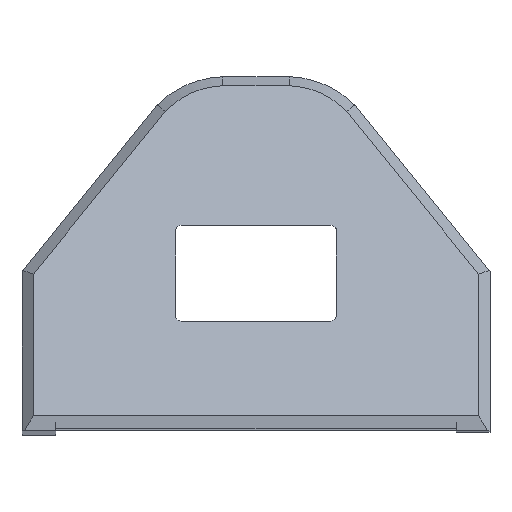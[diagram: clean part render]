
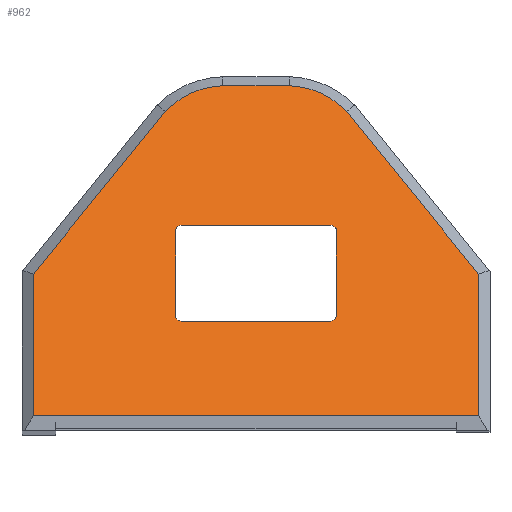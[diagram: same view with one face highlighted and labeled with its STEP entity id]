
A CAD part, top view. The second image highlights one B-rep face of the part: STEP entity #962.
In plain terms, the highlighted planar face has unit normal (0, 0.603, 0.798).
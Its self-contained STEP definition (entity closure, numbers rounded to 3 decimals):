
#20=FACE_BOUND('',#347,.T.);
#38=PLANE('',#1056);
#68=ELLIPSE('',#1057,0.626,0.5);
#69=ELLIPSE('',#1058,0.626,0.5);
#70=ELLIPSE('',#1059,0.626,0.5);
#71=ELLIPSE('',#1060,0.626,0.5);
#100=LINE('',#1491,#189);
#103=LINE('',#1498,#192);
#106=LINE('',#1529,#195);
#111=LINE('',#1589,#200);
#113=LINE('',#1665,#202);
#119=LINE('',#1677,#208);
#131=LINE('',#1705,#220);
#132=LINE('',#1709,#221);
#133=LINE('',#1713,#222);
#134=LINE('',#1717,#223);
#189=VECTOR('',#1193,10.);
#192=VECTOR('',#1198,10.);
#195=VECTOR('',#1205,10.);
#200=VECTOR('',#1212,10.);
#202=VECTOR('',#1216,10.);
#208=VECTOR('',#1228,10.);
#220=VECTOR('',#1252,10.);
#221=VECTOR('',#1255,10.);
#222=VECTOR('',#1258,10.);
#223=VECTOR('',#1261,10.);
#293=FACE_OUTER_BOUND('',#346,.T.);
#346=EDGE_LOOP('',(#794,#795,#796,#797,#798,#799,#800,#801));
#347=EDGE_LOOP('',(#802,#803,#804,#805,#806,#807,#808,#809));
#379=B_SPLINE_CURVE_WITH_KNOTS('',3,(#1558,#1559,#1560,#1561,#1562),
 .UNSPECIFIED.,.F.,.F.,(4,1,4),(-3.112,-2.672,-2.338),
 .UNSPECIFIED.);
#384=B_SPLINE_CURVE_WITH_KNOTS('',3,(#1626,#1627,#1628,#1629,#1630),
 .UNSPECIFIED.,.F.,.F.,(4,1,4),(2.338,2.783,3.112),
 .UNSPECIFIED.);
#446=VERTEX_POINT('',#1488);
#447=VERTEX_POINT('',#1490);
#449=VERTEX_POINT('',#1496);
#450=VERTEX_POINT('',#1497);
#454=VERTEX_POINT('',#1528);
#458=VERTEX_POINT('',#1557);
#461=VERTEX_POINT('',#1588);
#463=VERTEX_POINT('',#1625);
#477=VERTEX_POINT('',#1703);
#478=VERTEX_POINT('',#1704);
#479=VERTEX_POINT('',#1706);
#480=VERTEX_POINT('',#1708);
#481=VERTEX_POINT('',#1710);
#482=VERTEX_POINT('',#1712);
#483=VERTEX_POINT('',#1714);
#484=VERTEX_POINT('',#1716);
#554=EDGE_CURVE('',#446,#447,#100,.T.);
#557=EDGE_CURVE('',#449,#450,#103,.T.);
#562=EDGE_CURVE('',#450,#454,#106,.T.);
#567=EDGE_CURVE('',#458,#449,#379,.T.);
#571=EDGE_CURVE('',#461,#458,#111,.T.);
#574=EDGE_CURVE('',#463,#461,#384,.T.);
#578=EDGE_CURVE('',#447,#463,#113,.T.);
#585=EDGE_CURVE('',#454,#446,#119,.T.);
#598=EDGE_CURVE('',#477,#478,#131,.T.);
#599=EDGE_CURVE('',#478,#479,#68,.T.);
#600=EDGE_CURVE('',#479,#480,#132,.T.);
#601=EDGE_CURVE('',#480,#481,#69,.T.);
#602=EDGE_CURVE('',#481,#482,#133,.T.);
#603=EDGE_CURVE('',#482,#483,#70,.T.);
#604=EDGE_CURVE('',#483,#484,#134,.T.);
#605=EDGE_CURVE('',#484,#477,#71,.T.);
#794=ORIENTED_EDGE('',*,*,#554,.F.);
#795=ORIENTED_EDGE('',*,*,#585,.F.);
#796=ORIENTED_EDGE('',*,*,#562,.F.);
#797=ORIENTED_EDGE('',*,*,#557,.F.);
#798=ORIENTED_EDGE('',*,*,#567,.F.);
#799=ORIENTED_EDGE('',*,*,#571,.F.);
#800=ORIENTED_EDGE('',*,*,#574,.F.);
#801=ORIENTED_EDGE('',*,*,#578,.F.);
#802=ORIENTED_EDGE('',*,*,#598,.T.);
#803=ORIENTED_EDGE('',*,*,#599,.T.);
#804=ORIENTED_EDGE('',*,*,#600,.T.);
#805=ORIENTED_EDGE('',*,*,#601,.T.);
#806=ORIENTED_EDGE('',*,*,#602,.T.);
#807=ORIENTED_EDGE('',*,*,#603,.T.);
#808=ORIENTED_EDGE('',*,*,#604,.T.);
#809=ORIENTED_EDGE('',*,*,#605,.T.);
#962=ADVANCED_FACE('',(#293,#20),#38,.T.);
#1056=AXIS2_PLACEMENT_3D('',#1702,#1250,#1251);
#1057=AXIS2_PLACEMENT_3D('',#1707,#1253,#1254);
#1058=AXIS2_PLACEMENT_3D('',#1711,#1256,#1257);
#1059=AXIS2_PLACEMENT_3D('',#1715,#1259,#1260);
#1060=AXIS2_PLACEMENT_3D('',#1718,#1262,#1263);
#1193=DIRECTION('',(0.,0.798,-0.602));
#1198=DIRECTION('',(0.543,-0.67,0.506));
#1205=DIRECTION('',(0.,-0.798,0.602));
#1212=DIRECTION('',(1.,0.,0.));
#1216=DIRECTION('',(0.543,0.67,-0.506));
#1228=DIRECTION('',(-1.,0.,0.));
#1250=DIRECTION('center_axis',(0.,0.602,0.798));
#1251=DIRECTION('ref_axis',(1.,0.,0.));
#1252=DIRECTION('',(1.,0.,0.));
#1253=DIRECTION('center_axis',(0.,-0.602,-0.798));
#1254=DIRECTION('ref_axis',(0.,0.798,-0.602));
#1255=DIRECTION('',(0.,-0.798,0.602));
#1256=DIRECTION('center_axis',(0.,-0.602,-0.798));
#1257=DIRECTION('ref_axis',(0.,0.798,-0.602));
#1258=DIRECTION('',(-1.,0.,0.));
#1259=DIRECTION('center_axis',(0.,-0.602,-0.798));
#1260=DIRECTION('ref_axis',(0.,-0.798,0.602));
#1261=DIRECTION('',(0.,0.798,-0.602));
#1262=DIRECTION('center_axis',(0.,-0.602,-0.798));
#1263=DIRECTION('ref_axis',(0.,-0.798,0.602));
#1488=CARTESIAN_POINT('',(-19.715,1.009,256.8));
#1490=CARTESIAN_POINT('',(-19.715,13.564,247.323));
#1491=CARTESIAN_POINT('',(-19.715,68.818,205.612));
#1496=CARTESIAN_POINT('',(8.037,27.981,236.439));
#1497=CARTESIAN_POINT('',(19.715,13.564,247.323));
#1498=CARTESIAN_POINT('',(-19.426,61.884,210.846));
#1528=CARTESIAN_POINT('',(19.715,1.009,256.8));
#1529=CARTESIAN_POINT('',(19.715,68.818,205.612));
#1557=CARTESIAN_POINT('',(2.934,30.262,234.717));
#1558=CARTESIAN_POINT('Ctrl Pts',(2.934,30.262,234.717));
#1559=CARTESIAN_POINT('Ctrl Pts',(3.995,30.23,234.741));
#1560=CARTESIAN_POINT('Ctrl Pts',(5.856,29.761,235.096));
#1561=CARTESIAN_POINT('Ctrl Pts',(7.446,28.592,235.978));
#1562=CARTESIAN_POINT('Ctrl Pts',(8.037,27.981,236.439));
#1588=CARTESIAN_POINT('',(-2.934,30.262,234.717));
#1589=CARTESIAN_POINT('',(-3.703,30.262,234.717));
#1625=CARTESIAN_POINT('',(-8.037,27.981,236.439));
#1626=CARTESIAN_POINT('Ctrl Pts',(-8.037,27.981,236.439));
#1627=CARTESIAN_POINT('Ctrl Pts',(-7.25,28.796,235.824));
#1628=CARTESIAN_POINT('Ctrl Pts',(-5.588,29.877,235.008));
#1629=CARTESIAN_POINT('Ctrl Pts',(-3.726,30.238,234.735));
#1630=CARTESIAN_POINT('Ctrl Pts',(-2.934,30.262,234.717));
#1665=CARTESIAN_POINT('',(16.373,58.115,213.692));
#1677=CARTESIAN_POINT('',(5.179,1.009,256.8));
#1702=CARTESIAN_POINT('Origin',(-10.358,16.518,245.093));
#1703=CARTESIAN_POINT('',(-6.619,17.906,244.045));
#1704=CARTESIAN_POINT('',(6.619,17.906,244.045));
#1705=CARTESIAN_POINT('',(-1.869,17.906,244.045));
#1706=CARTESIAN_POINT('',(7.119,17.406,244.422));
#1707=CARTESIAN_POINT('Origin',(6.619,17.406,244.422));
#1708=CARTESIAN_POINT('',(7.119,9.906,250.084));
#1709=CARTESIAN_POINT('',(7.119,68.652,205.737));
#1710=CARTESIAN_POINT('',(6.619,9.406,250.461));
#1711=CARTESIAN_POINT('Origin',(6.619,9.906,250.084));
#1712=CARTESIAN_POINT('',(-6.619,9.406,250.461));
#1713=CARTESIAN_POINT('',(-8.488,9.406,250.461));
#1714=CARTESIAN_POINT('',(-7.119,9.906,250.084));
#1715=CARTESIAN_POINT('Origin',(-6.619,9.906,250.084));
#1716=CARTESIAN_POINT('',(-7.119,17.406,244.422));
#1717=CARTESIAN_POINT('',(-7.119,71.041,203.934));
#1718=CARTESIAN_POINT('Origin',(-6.619,17.406,244.422));
